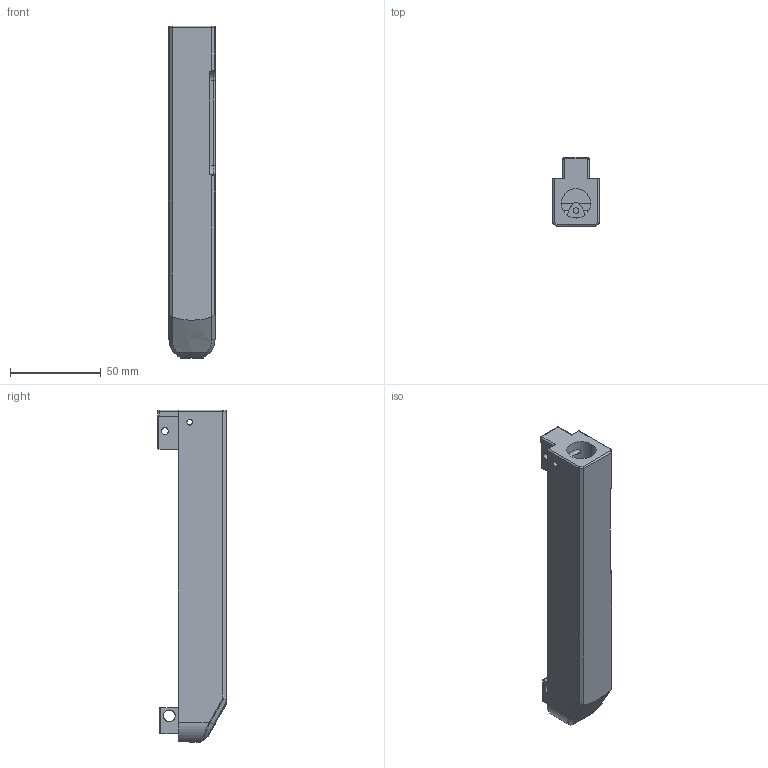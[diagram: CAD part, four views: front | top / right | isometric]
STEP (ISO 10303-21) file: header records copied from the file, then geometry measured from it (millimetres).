
FILE_DESCRIPTION (( 'STEP AP214' ), '1' );
FILE_NAME ('Merlin 795 release no rail.STEP', '2021-07-15T18:07:40', ( 'RJ' ), ( '' ), 'SwSTEP 2.0', 'SolidWorks 2015', '' );
FILE_SCHEMA (( 'AUTOMOTIVE_DESIGN' ));
Length unit declared in the file: millimetre
Products named in the file (1): Merlin 795 release no rail
Bounding box: 25.5 x 38 x 183 mm (x, y, z)
Volume: 56707.5 mm3; surface area: 27704.9 mm2
Topology: 1 solids, 1 shells, 129 faces, 342 edges, 215 vertices
Faces by surface type: plane 53, cylinder 48, bspline 24, torus 4
Entity records: 5443 total; most frequent: CARTESIAN_POINT 2406, ORIENTED_EDGE 684, DIRECTION 533, EDGE_CURVE 342, VERTEX_POINT 215, LINE 193, VECTOR 193, AXIS2_PLACEMENT_3D 170
